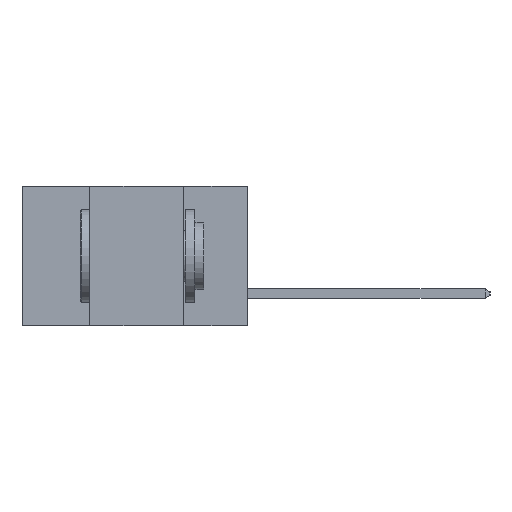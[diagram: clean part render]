
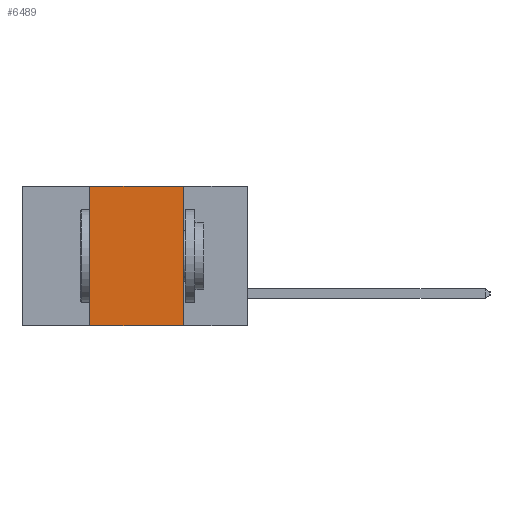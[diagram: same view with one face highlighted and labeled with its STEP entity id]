
A CAD part, left-side view. The second image highlights one B-rep face of the part: STEP entity #6489.
In plain terms, the highlighted planar face has unit normal (-1, 0, 0).
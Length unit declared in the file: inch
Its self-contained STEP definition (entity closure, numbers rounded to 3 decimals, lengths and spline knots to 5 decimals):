
#590 = LINE ( 'NONE', #12118, #7186 ) ;
#865 = EDGE_CURVE ( 'NONE', #11633, #9889, #2197, .T. ) ;
#2197 = LINE ( 'NONE', #6800, #16081 ) ;
#2647 = EDGE_LOOP ( 'NONE', ( #7291, #16742, #4236, #6462 ) ) ;
#2705 = CARTESIAN_POINT ( 'NONE',  ( 0., 0.42, 0. ) ) ;
#3715 = EDGE_CURVE ( 'NONE', #3957, #9808, #12311, .T. ) ;
#3957 = VERTEX_POINT ( 'NONE', #15648 ) ;
#4236 = ORIENTED_EDGE ( 'NONE', *, *, #3715, .F. ) ;
#6101 = DIRECTION ( 'NONE',  ( 0., 0., 1. ) ) ;
#6210 = EDGE_CURVE ( 'NONE', #9808, #11633, #15119, .T. ) ;
#6462 = ORIENTED_EDGE ( 'NONE', *, *, #8784, .T. ) ;
#6489 = ADVANCED_FACE ( 'NONE', ( #10414 ), #16723, .F. ) ;
#6800 = CARTESIAN_POINT ( 'NONE',  ( 0., 0.17, 0. ) ) ;
#7186 = VECTOR ( 'NONE', #12048, 39.37008 ) ;
#7291 = ORIENTED_EDGE ( 'NONE', *, *, #865, .F. ) ;
#7870 = CARTESIAN_POINT ( 'NONE',  ( 0., 0.42, 0. ) ) ;
#8676 = VECTOR ( 'NONE', #6101, 39.37008 ) ;
#8784 = EDGE_CURVE ( 'NONE', #3957, #9889, #590, .T. ) ;
#9112 = DIRECTION ( 'NONE',  ( 0., -1., 0. ) ) ;
#9808 = VERTEX_POINT ( 'NONE', #7870 ) ;
#9889 = VERTEX_POINT ( 'NONE', #12111 ) ;
#10414 = FACE_OUTER_BOUND ( 'NONE', #2647, .T. ) ;
#10426 = CARTESIAN_POINT ( 'NONE',  ( 0., 0.6, 0. ) ) ;
#10442 = CARTESIAN_POINT ( 'NONE',  ( 0., 0.17, 0. ) ) ;
#11476 = VECTOR ( 'NONE', #9112, 39.37008 ) ;
#11633 = VERTEX_POINT ( 'NONE', #10442 ) ;
#12048 = DIRECTION ( 'NONE',  ( 0., -1., 0. ) ) ;
#12111 = CARTESIAN_POINT ( 'NONE',  ( 0., 0.17, -0.37 ) ) ;
#12118 = CARTESIAN_POINT ( 'NONE',  ( 0., 0.6, -0.37 ) ) ;
#12311 = LINE ( 'NONE', #2705, #8676 ) ;
#13126 = AXIS2_PLACEMENT_3D ( 'NONE', #16324, #16308, #16242 ) ;
#15119 = LINE ( 'NONE', #10426, #11476 ) ;
#15648 = CARTESIAN_POINT ( 'NONE',  ( 0., 0.42, -0.37 ) ) ;
#16081 = VECTOR ( 'NONE', #16204, 39.37008 ) ;
#16204 = DIRECTION ( 'NONE',  ( 0., 0., -1. ) ) ;
#16242 = DIRECTION ( 'NONE',  ( 0., 0., -1. ) ) ;
#16308 = DIRECTION ( 'NONE',  ( 1., 0., 0. ) ) ;
#16324 = CARTESIAN_POINT ( 'NONE',  ( 0., 0.6, 0. ) ) ;
#16723 = PLANE ( 'NONE',  #13126 ) ;
#16742 = ORIENTED_EDGE ( 'NONE', *, *, #6210, .F. ) ;
